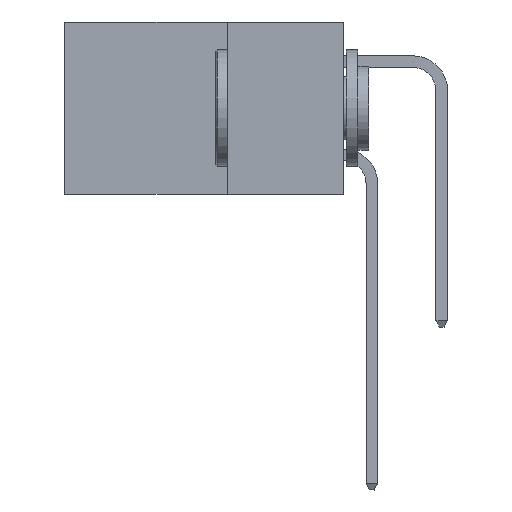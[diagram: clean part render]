
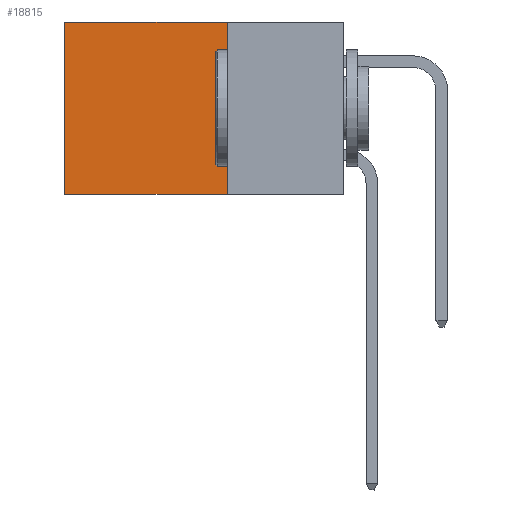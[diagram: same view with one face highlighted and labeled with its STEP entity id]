
A CAD part, left-side view. The second image highlights one B-rep face of the part: STEP entity #18815.
In plain terms, the highlighted planar face has unit normal (-1, 0, 0).
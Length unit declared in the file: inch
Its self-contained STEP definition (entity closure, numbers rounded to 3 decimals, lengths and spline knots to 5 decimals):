
#568 = DIRECTION ( 'NONE',  ( 0., 0., -1. ) ) ;
#973 = DIRECTION ( 'NONE',  ( 0., 0., -1. ) ) ;
#1875 = CARTESIAN_POINT ( 'NONE',  ( 0.298, 0.6, -0.37 ) ) ;
#3363 = CARTESIAN_POINT ( 'NONE',  ( 0.298, 0.25, -0.37 ) ) ;
#4854 = VECTOR ( 'NONE', #7521, 39.37008 ) ;
#5223 = LINE ( 'NONE', #18273, #8656 ) ;
#5513 = CARTESIAN_POINT ( 'NONE',  ( 0.298, 0.25, 0. ) ) ;
#5646 = ORIENTED_EDGE ( 'NONE', *, *, #11790, .T. ) ;
#5720 = EDGE_CURVE ( 'NONE', #16191, #7229, #21156, .T. ) ;
#6090 = VECTOR ( 'NONE', #973, 39.37008 ) ;
#6105 = CARTESIAN_POINT ( 'NONE',  ( 0.298, 0.25, 0. ) ) ;
#6250 = DIRECTION ( 'NONE',  ( 0., 1., 0. ) ) ;
#6878 = CARTESIAN_POINT ( 'NONE',  ( 0.298, 0.25, 0. ) ) ;
#7229 = VERTEX_POINT ( 'NONE', #1875 ) ;
#7411 = VECTOR ( 'NONE', #6250, 39.37008 ) ;
#7521 = DIRECTION ( 'NONE',  ( 0., 1., 0. ) ) ;
#8107 = DIRECTION ( 'NONE',  ( 0., 0., -1. ) ) ;
#8656 = VECTOR ( 'NONE', #568, 39.37008 ) ;
#8708 = AXIS2_PLACEMENT_3D ( 'NONE', #6105, #19820, #8107 ) ;
#8938 = VERTEX_POINT ( 'NONE', #6878 ) ;
#8991 = CARTESIAN_POINT ( 'NONE',  ( 0.298, 0.6, 0. ) ) ;
#10215 = CARTESIAN_POINT ( 'NONE',  ( 0.298, 0.25, -0.37 ) ) ;
#11790 = EDGE_CURVE ( 'NONE', #14414, #7229, #21085, .T. ) ;
#12845 = CARTESIAN_POINT ( 'NONE',  ( 0.298, 0.6, 0. ) ) ;
#13601 = ORIENTED_EDGE ( 'NONE', *, *, #5720, .F. ) ;
#13964 = EDGE_LOOP ( 'NONE', ( #5646, #13601, #23187, #22853 ) ) ;
#14414 = VERTEX_POINT ( 'NONE', #8991 ) ;
#15321 = LINE ( 'NONE', #5513, #4854 ) ;
#16191 = VERTEX_POINT ( 'NONE', #10215 ) ;
#18273 = CARTESIAN_POINT ( 'NONE',  ( 0.298, 0.25, 0. ) ) ;
#18815 = ADVANCED_FACE ( 'NONE', ( #20723 ), #21661, .F. ) ;
#19630 = EDGE_CURVE ( 'NONE', #8938, #16191, #5223, .T. ) ;
#19820 = DIRECTION ( 'NONE',  ( 1., 0., 0. ) ) ;
#20721 = EDGE_CURVE ( 'NONE', #8938, #14414, #15321, .T. ) ;
#20723 = FACE_OUTER_BOUND ( 'NONE', #13964, .T. ) ;
#21085 = LINE ( 'NONE', #12845, #6090 ) ;
#21156 = LINE ( 'NONE', #3363, #7411 ) ;
#21661 = PLANE ( 'NONE',  #8708 ) ;
#22853 = ORIENTED_EDGE ( 'NONE', *, *, #20721, .T. ) ;
#23187 = ORIENTED_EDGE ( 'NONE', *, *, #19630, .F. ) ;
